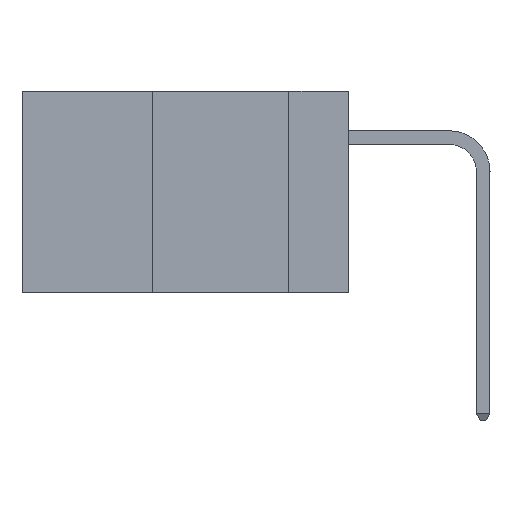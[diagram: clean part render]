
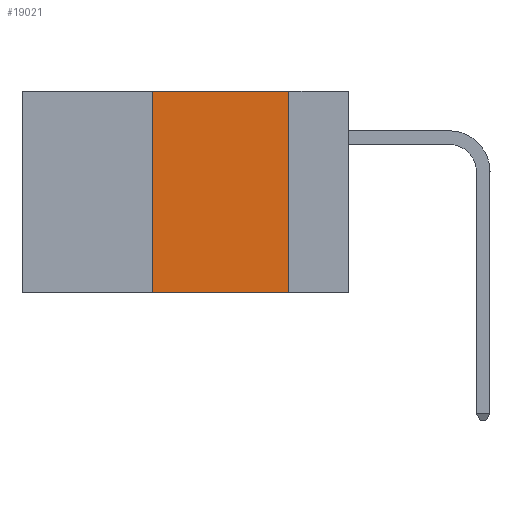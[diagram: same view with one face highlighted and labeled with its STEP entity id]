
A CAD part, left-side view. The second image highlights one B-rep face of the part: STEP entity #19021.
In plain terms, the highlighted planar face has unit normal (-1, 0, 0).
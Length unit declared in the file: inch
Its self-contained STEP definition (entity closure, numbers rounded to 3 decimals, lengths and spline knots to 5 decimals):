
#1114 = VERTEX_POINT ( 'NONE', #16525 ) ;
#3629 = EDGE_CURVE ( 'NONE', #20731, #1114, #40054, .T. ) ;
#4775 = DIRECTION ( 'NONE',  ( 0., 0., 1. ) ) ;
#5043 = DIRECTION ( 'NONE',  ( 0., -1., 0. ) ) ;
#5357 = PLANE ( 'NONE',  #42889 ) ;
#5623 = VERTEX_POINT ( 'NONE', #15234 ) ;
#5697 = VECTOR ( 'NONE', #5043, 39.37008 ) ;
#10105 = CARTESIAN_POINT ( 'NONE',  ( 0., 0.11, 0. ) ) ;
#11467 = ORIENTED_EDGE ( 'NONE', *, *, #29953, .T. ) ;
#12649 = LINE ( 'NONE', #25735, #5697 ) ;
#12969 = CARTESIAN_POINT ( 'NONE',  ( 0., 0.11, 0. ) ) ;
#15234 = CARTESIAN_POINT ( 'NONE',  ( 0., 0.11, -0.37 ) ) ;
#15703 = DIRECTION ( 'NONE',  ( 1., 0., 0. ) ) ;
#15763 = ORIENTED_EDGE ( 'NONE', *, *, #41646, .F. ) ;
#16525 = CARTESIAN_POINT ( 'NONE',  ( 0., 0.36, 0. ) ) ;
#16575 = VECTOR ( 'NONE', #34462, 39.37008 ) ;
#16617 = EDGE_CURVE ( 'NONE', #1114, #39754, #23301, .T. ) ;
#17377 = ORIENTED_EDGE ( 'NONE', *, *, #3629, .F. ) ;
#17671 = LINE ( 'NONE', #10105, #16575 ) ;
#19021 = ADVANCED_FACE ( 'NONE', ( #28677 ), #5357, .F. ) ;
#20731 = VERTEX_POINT ( 'NONE', #23813 ) ;
#21958 = CARTESIAN_POINT ( 'NONE',  ( 0., 0.36, 0. ) ) ;
#22200 = VECTOR ( 'NONE', #37847, 39.37008 ) ;
#23301 = LINE ( 'NONE', #27439, #22200 ) ;
#23813 = CARTESIAN_POINT ( 'NONE',  ( 0., 0.36, -0.37 ) ) ;
#24460 = EDGE_LOOP ( 'NONE', ( #15763, #30864, #17377, #11467 ) ) ;
#25735 = CARTESIAN_POINT ( 'NONE',  ( 0., 0.6, -0.37 ) ) ;
#27439 = CARTESIAN_POINT ( 'NONE',  ( 0., 0.6, 0. ) ) ;
#28677 = FACE_OUTER_BOUND ( 'NONE', #24460, .T. ) ;
#29953 = EDGE_CURVE ( 'NONE', #20731, #5623, #12649, .T. ) ;
#30864 = ORIENTED_EDGE ( 'NONE', *, *, #16617, .F. ) ;
#33002 = VECTOR ( 'NONE', #4775, 39.37008 ) ;
#34462 = DIRECTION ( 'NONE',  ( 0., 0., -1. ) ) ;
#36635 = CARTESIAN_POINT ( 'NONE',  ( 0., 0.6, 0. ) ) ;
#37847 = DIRECTION ( 'NONE',  ( 0., -1., 0. ) ) ;
#39754 = VERTEX_POINT ( 'NONE', #12969 ) ;
#40054 = LINE ( 'NONE', #21958, #33002 ) ;
#40093 = DIRECTION ( 'NONE',  ( 0., 0., -1. ) ) ;
#41646 = EDGE_CURVE ( 'NONE', #39754, #5623, #17671, .T. ) ;
#42889 = AXIS2_PLACEMENT_3D ( 'NONE', #36635, #15703, #40093 ) ;
